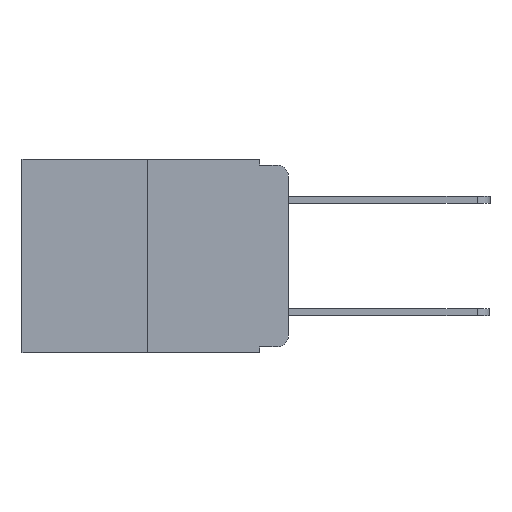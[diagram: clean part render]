
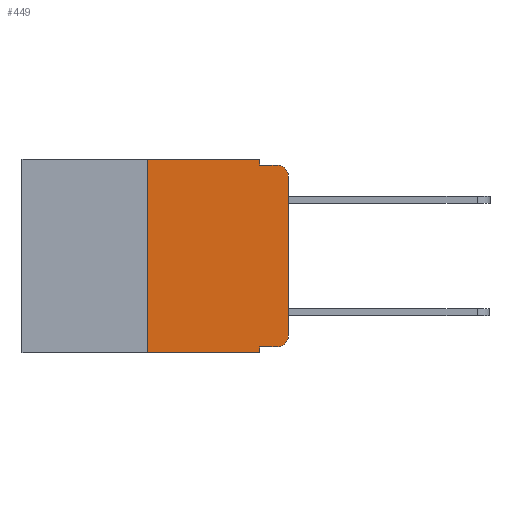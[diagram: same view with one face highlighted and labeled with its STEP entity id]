
A CAD part, left-side view. The second image highlights one B-rep face of the part: STEP entity #449.
In plain terms, the highlighted planar face has unit normal (-1, 0, 0).
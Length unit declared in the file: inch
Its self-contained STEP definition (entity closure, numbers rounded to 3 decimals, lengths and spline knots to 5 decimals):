
#49 = AXIS2_PLACEMENT_3D ( 'NONE', #1789, #7267, #2766 ) ;
#55 = LINE ( 'NONE', #4785, #6763 ) ;
#235 = LINE ( 'NONE', #1160, #4667 ) ;
#424 = CARTESIAN_POINT ( 'NONE',  ( 0., 0.02, -0.01 ) ) ;
#449 = ADVANCED_FACE ( 'NONE', ( #7773 ), #838, .F. ) ;
#743 = VERTEX_POINT ( 'NONE', #8991 ) ;
#772 = EDGE_LOOP ( 'NONE', ( #3725, #2162, #2535, #7145, #1082, #4161, #1206, #3123, #3615, #4066 ) ) ;
#778 = DIRECTION ( 'NONE',  ( 0., -1., 0. ) ) ;
#838 = PLANE ( 'NONE',  #2417 ) ;
#840 = EDGE_CURVE ( 'NONE', #1659, #9355, #9833, .T. ) ;
#939 = EDGE_CURVE ( 'NONE', #2634, #9355, #235, .T. ) ;
#1082 = ORIENTED_EDGE ( 'NONE', *, *, #2620, .F. ) ;
#1160 = CARTESIAN_POINT ( 'NONE',  ( 0., 0.473, -0.343 ) ) ;
#1206 = ORIENTED_EDGE ( 'NONE', *, *, #939, .T. ) ;
#1235 = EDGE_CURVE ( 'NONE', #3991, #4293, #4325, .T. ) ;
#1327 = VECTOR ( 'NONE', #1866, 39.37008 ) ;
#1475 = DIRECTION ( 'NONE',  ( 0., 0., -1. ) ) ;
#1488 = CARTESIAN_POINT ( 'NONE',  ( 0., 0.051, 0. ) ) ;
#1631 = DIRECTION ( 'NONE',  ( 1., 0., 0. ) ) ;
#1659 = VERTEX_POINT ( 'NONE', #3901 ) ;
#1789 = CARTESIAN_POINT ( 'NONE',  ( 0., 0.02, -0.03 ) ) ;
#1866 = DIRECTION ( 'NONE',  ( 0., -1., 0. ) ) ;
#1880 = CARTESIAN_POINT ( 'NONE',  ( 0., 0.051, -0.333 ) ) ;
#2100 = VERTEX_POINT ( 'NONE', #5459 ) ;
#2120 = VECTOR ( 'NONE', #4700, 39.37008 ) ;
#2162 = ORIENTED_EDGE ( 'NONE', *, *, #8266, .T. ) ;
#2417 = AXIS2_PLACEMENT_3D ( 'NONE', #8272, #1631, #1475 ) ;
#2487 = DIRECTION ( 'NONE',  ( 0., 0., -1. ) ) ;
#2526 = AXIS2_PLACEMENT_3D ( 'NONE', #6744, #6375, #8116 ) ;
#2535 = ORIENTED_EDGE ( 'NONE', *, *, #1235, .F. ) ;
#2620 = EDGE_CURVE ( 'NONE', #4431, #7090, #55, .T. ) ;
#2634 = VERTEX_POINT ( 'NONE', #4447 ) ;
#2766 = DIRECTION ( 'NONE',  ( 0., 0., -1. ) ) ;
#2863 = CARTESIAN_POINT ( 'NONE',  ( 0., 0.02, -0.333 ) ) ;
#3013 = EDGE_CURVE ( 'NONE', #1659, #6895, #5721, .T. ) ;
#3123 = ORIENTED_EDGE ( 'NONE', *, *, #840, .F. ) ;
#3158 = DIRECTION ( 'NONE',  ( 0., 0., -1. ) ) ;
#3233 = CARTESIAN_POINT ( 'NONE',  ( 0., 0.051, 0. ) ) ;
#3281 = DIRECTION ( 'NONE',  ( 0., 0., 1. ) ) ;
#3494 = DIRECTION ( 'NONE',  ( 0., -1., 0. ) ) ;
#3615 = ORIENTED_EDGE ( 'NONE', *, *, #3013, .T. ) ;
#3725 = ORIENTED_EDGE ( 'NONE', *, *, #4072, .T. ) ;
#3779 = VECTOR ( 'NONE', #2487, 39.37008 ) ;
#3901 = CARTESIAN_POINT ( 'NONE',  ( 0., 0.051, -0.333 ) ) ;
#3932 = VECTOR ( 'NONE', #6073, 39.37008 ) ;
#3991 = VERTEX_POINT ( 'NONE', #7496 ) ;
#4027 = LINE ( 'NONE', #1488, #3779 ) ;
#4066 = ORIENTED_EDGE ( 'NONE', *, *, #4134, .T. ) ;
#4072 = EDGE_CURVE ( 'NONE', #2100, #743, #5705, .T. ) ;
#4134 = EDGE_CURVE ( 'NONE', #6895, #2100, #8605, .T. ) ;
#4161 = ORIENTED_EDGE ( 'NONE', *, *, #4552, .F. ) ;
#4189 = LINE ( 'NONE', #9072, #3932 ) ;
#4256 = CARTESIAN_POINT ( 'NONE',  ( 0., 0., 0. ) ) ;
#4293 = VERTEX_POINT ( 'NONE', #424 ) ;
#4325 = LINE ( 'NONE', #10083, #2120 ) ;
#4431 = VERTEX_POINT ( 'NONE', #9103 ) ;
#4447 = CARTESIAN_POINT ( 'NONE',  ( 0., 0.25, -0.343 ) ) ;
#4552 = EDGE_CURVE ( 'NONE', #2634, #4431, #4189, .T. ) ;
#4667 = VECTOR ( 'NONE', #778, 39.37008 ) ;
#4700 = DIRECTION ( 'NONE',  ( 0., -1., 0. ) ) ;
#4785 = CARTESIAN_POINT ( 'NONE',  ( 0., 0.473, 0. ) ) ;
#5378 = CARTESIAN_POINT ( 'NONE',  ( 0., 0.051, 0. ) ) ;
#5459 = CARTESIAN_POINT ( 'NONE',  ( 0., 0., -0.313 ) ) ;
#5614 = VECTOR ( 'NONE', #3158, 39.37008 ) ;
#5705 = LINE ( 'NONE', #4256, #9033 ) ;
#5721 = LINE ( 'NONE', #1880, #1327 ) ;
#6073 = DIRECTION ( 'NONE',  ( 0., 0., 1. ) ) ;
#6375 = DIRECTION ( 'NONE',  ( -1., 0., 0. ) ) ;
#6744 = CARTESIAN_POINT ( 'NONE',  ( 0., 0.02, -0.313 ) ) ;
#6763 = VECTOR ( 'NONE', #3494, 39.37008 ) ;
#6814 = CIRCLE ( 'NONE', #49, 0.02 ) ;
#6895 = VERTEX_POINT ( 'NONE', #2863 ) ;
#7090 = VERTEX_POINT ( 'NONE', #5378 ) ;
#7145 = ORIENTED_EDGE ( 'NONE', *, *, #8087, .F. ) ;
#7267 = DIRECTION ( 'NONE',  ( -1., 0., 0. ) ) ;
#7496 = CARTESIAN_POINT ( 'NONE',  ( 0., 0.051, -0.01 ) ) ;
#7773 = FACE_OUTER_BOUND ( 'NONE', #772, .T. ) ;
#8087 = EDGE_CURVE ( 'NONE', #7090, #3991, #4027, .T. ) ;
#8116 = DIRECTION ( 'NONE',  ( 0., 0., -1. ) ) ;
#8266 = EDGE_CURVE ( 'NONE', #743, #4293, #6814, .T. ) ;
#8272 = CARTESIAN_POINT ( 'NONE',  ( 0., 0.473, 0. ) ) ;
#8605 = CIRCLE ( 'NONE', #2526, 0.02 ) ;
#8991 = CARTESIAN_POINT ( 'NONE',  ( 0., 0., -0.03 ) ) ;
#9033 = VECTOR ( 'NONE', #3281, 39.37008 ) ;
#9072 = CARTESIAN_POINT ( 'NONE',  ( 0., 0.25, 0. ) ) ;
#9103 = CARTESIAN_POINT ( 'NONE',  ( 0., 0.25, 0. ) ) ;
#9355 = VERTEX_POINT ( 'NONE', #10113 ) ;
#9833 = LINE ( 'NONE', #3233, #5614 ) ;
#10083 = CARTESIAN_POINT ( 'NONE',  ( 0., 0.051, -0.01 ) ) ;
#10113 = CARTESIAN_POINT ( 'NONE',  ( 0., 0.051, -0.343 ) ) ;
